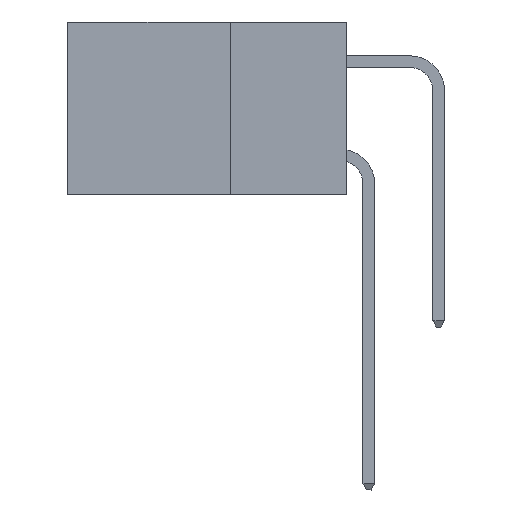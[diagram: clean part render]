
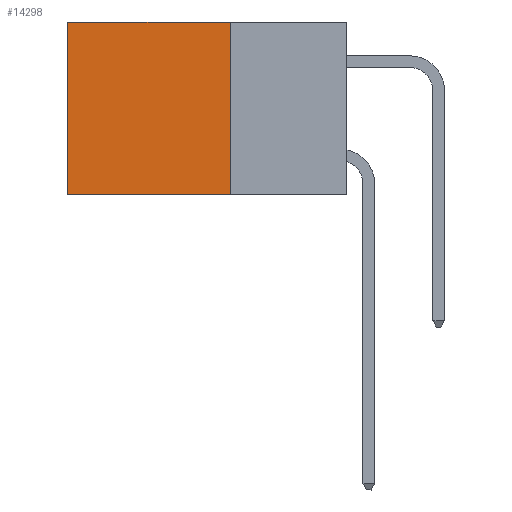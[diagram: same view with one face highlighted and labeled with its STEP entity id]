
A CAD part, left-side view. The second image highlights one B-rep face of the part: STEP entity #14298.
In plain terms, the highlighted planar face has unit normal (-1, 0, 0).
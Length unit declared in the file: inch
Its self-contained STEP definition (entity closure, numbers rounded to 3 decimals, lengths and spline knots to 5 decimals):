
#781 = CARTESIAN_POINT ( 'NONE',  ( 0.2875, 0.25, 0. ) ) ;
#2791 = ORIENTED_EDGE ( 'NONE', *, *, #19830, .T. ) ;
#3299 = CARTESIAN_POINT ( 'NONE',  ( 0.2875, 0.25, -0.37 ) ) ;
#3520 = CARTESIAN_POINT ( 'NONE',  ( 0.2875, 0.6, 0. ) ) ;
#4023 = CARTESIAN_POINT ( 'NONE',  ( 0.2875, 0.25, -0.37 ) ) ;
#4157 = FACE_OUTER_BOUND ( 'NONE', #6158, .T. ) ;
#4580 = DIRECTION ( 'NONE',  ( 0., 1., 0. ) ) ;
#5019 = ORIENTED_EDGE ( 'NONE', *, *, #22211, .F. ) ;
#5399 = DIRECTION ( 'NONE',  ( 0., 1., 0. ) ) ;
#5517 = ORIENTED_EDGE ( 'NONE', *, *, #22505, .T. ) ;
#6158 = EDGE_LOOP ( 'NONE', ( #2791, #22626, #5019, #5517 ) ) ;
#6292 = LINE ( 'NONE', #20092, #13463 ) ;
#6353 = VECTOR ( 'NONE', #4580, 39.37008 ) ;
#8511 = VERTEX_POINT ( 'NONE', #12148 ) ;
#11631 = VECTOR ( 'NONE', #12117, 39.37008 ) ;
#12117 = DIRECTION ( 'NONE',  ( 0., 0., -1. ) ) ;
#12148 = CARTESIAN_POINT ( 'NONE',  ( 0.2875, 0.6, -0.37 ) ) ;
#12575 = PLANE ( 'NONE',  #20289 ) ;
#13463 = VECTOR ( 'NONE', #17849, 39.37008 ) ;
#14298 = ADVANCED_FACE ( 'NONE', ( #4157 ), #12575, .F. ) ;
#14320 = CARTESIAN_POINT ( 'NONE',  ( 0.2875, 0.6, 0. ) ) ;
#16223 = VERTEX_POINT ( 'NONE', #20266 ) ;
#16404 = EDGE_CURVE ( 'NONE', #20088, #8511, #18689, .T. ) ;
#17030 = VERTEX_POINT ( 'NONE', #3520 ) ;
#17849 = DIRECTION ( 'NONE',  ( 0., 0., -1. ) ) ;
#18689 = LINE ( 'NONE', #3299, #21206 ) ;
#19830 = EDGE_CURVE ( 'NONE', #17030, #8511, #22338, .T. ) ;
#20088 = VERTEX_POINT ( 'NONE', #4023 ) ;
#20092 = CARTESIAN_POINT ( 'NONE',  ( 0.2875, 0.25, 0. ) ) ;
#20266 = CARTESIAN_POINT ( 'NONE',  ( 0.2875, 0.25, 0. ) ) ;
#20289 = AXIS2_PLACEMENT_3D ( 'NONE', #20580, #24151, #20454 ) ;
#20454 = DIRECTION ( 'NONE',  ( 0., 0., -1. ) ) ;
#20580 = CARTESIAN_POINT ( 'NONE',  ( 0.2875, 0.25, 0. ) ) ;
#21206 = VECTOR ( 'NONE', #5399, 39.37008 ) ;
#22211 = EDGE_CURVE ( 'NONE', #16223, #20088, #6292, .T. ) ;
#22338 = LINE ( 'NONE', #14320, #11631 ) ;
#22505 = EDGE_CURVE ( 'NONE', #16223, #17030, #22971, .T. ) ;
#22626 = ORIENTED_EDGE ( 'NONE', *, *, #16404, .F. ) ;
#22971 = LINE ( 'NONE', #781, #6353 ) ;
#24151 = DIRECTION ( 'NONE',  ( 1., 0., 0. ) ) ;
